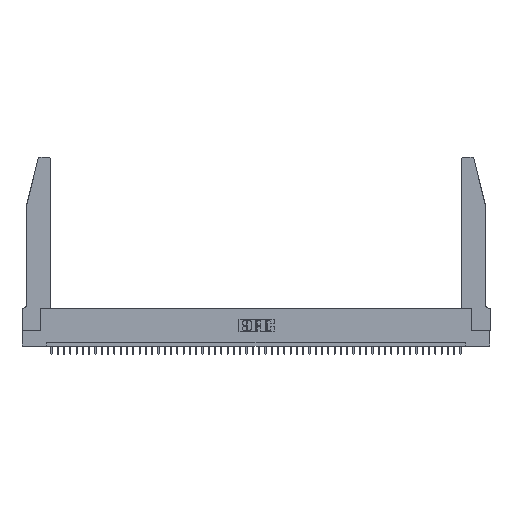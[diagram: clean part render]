
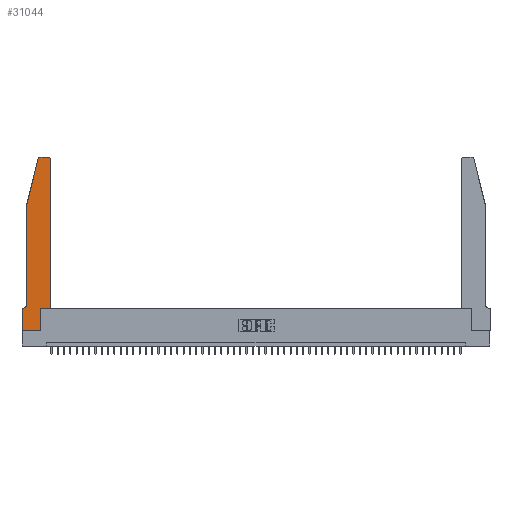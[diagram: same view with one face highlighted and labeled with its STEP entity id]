
A CAD part, top view. The second image highlights one B-rep face of the part: STEP entity #31044.
In plain terms, the highlighted planar face has unit normal (0, 0, 1).
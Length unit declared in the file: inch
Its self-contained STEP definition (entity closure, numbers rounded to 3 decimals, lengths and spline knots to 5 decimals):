
#136 = VERTEX_POINT ( 'NONE', #31626 ) ;
#412 = VECTOR ( 'NONE', #20663, 39.37008 ) ;
#1037 = ORIENTED_EDGE ( 'NONE', *, *, #36609, .T. ) ;
#2415 = CIRCLE ( 'NONE', #15642, 0.03 ) ;
#2477 = EDGE_CURVE ( 'NONE', #19180, #43705, #2415, .T. ) ;
#3498 = EDGE_LOOP ( 'NONE', ( #10704, #37596, #16229, #47534, #1037, #28264, #11088, #27232, #42411, #10031, #17437, #9026 ) ) ;
#3518 = LINE ( 'NONE', #20372, #21099 ) ;
#3726 = VERTEX_POINT ( 'NONE', #45273 ) ;
#4019 = DIRECTION ( 'NONE',  ( 0., -1., 0. ) ) ;
#5453 = AXIS2_PLACEMENT_3D ( 'NONE', #41027, #13496, #17654 ) ;
#7400 = CARTESIAN_POINT ( 'NONE',  ( 0.4505, 0.35, 0.37 ) ) ;
#7925 = DIRECTION ( 'NONE',  ( 0., 0., -1. ) ) ;
#8018 = VECTOR ( 'NONE', #47692, 39.37008 ) ;
#8240 = VERTEX_POINT ( 'NONE', #17943 ) ;
#8270 = CARTESIAN_POINT ( 'NONE',  ( 0.2865, 0.35, 0.37 ) ) ;
#8286 = DIRECTION ( 'NONE',  ( 1., 0., 0. ) ) ;
#8800 = VECTOR ( 'NONE', #20090, 39.37008 ) ;
#9026 = ORIENTED_EDGE ( 'NONE', *, *, #2477, .T. ) ;
#10031 = ORIENTED_EDGE ( 'NONE', *, *, #48210, .T. ) ;
#10631 = CARTESIAN_POINT ( 'NONE',  ( 0.0755, 0.42, 0.37 ) ) ;
#10704 = ORIENTED_EDGE ( 'NONE', *, *, #20610, .T. ) ;
#10705 = CARTESIAN_POINT ( 'NONE',  ( 0.2605, 2.75, 0.37 ) ) ;
#10942 = DIRECTION ( 'NONE',  ( -1., 0., 0. ) ) ;
#10972 = LINE ( 'NONE', #39771, #17835 ) ;
#11088 = ORIENTED_EDGE ( 'NONE', *, *, #26954, .T. ) ;
#11228 = DIRECTION ( 'NONE',  ( 1., 0., 0. ) ) ;
#12204 = AXIS2_PLACEMENT_3D ( 'NONE', #19861, #7925, #39593 ) ;
#13496 = DIRECTION ( 'NONE',  ( 0., 0., 1. ) ) ;
#15642 = AXIS2_PLACEMENT_3D ( 'NONE', #43852, #39432, #8286 ) ;
#15926 = CARTESIAN_POINT ( 'NONE',  ( 0., 0., 0.37 ) ) ;
#16121 = CARTESIAN_POINT ( 'NONE',  ( 0.0755, 2., 0.37 ) ) ;
#16218 = CARTESIAN_POINT ( 'NONE',  ( 0., 0., 0.37 ) ) ;
#16229 = ORIENTED_EDGE ( 'NONE', *, *, #16728, .T. ) ;
#16335 = CARTESIAN_POINT ( 'NONE',  ( 0.284, 2.72, 0.37 ) ) ;
#16728 = EDGE_CURVE ( 'NONE', #136, #44213, #35854, .T. ) ;
#17437 = ORIENTED_EDGE ( 'NONE', *, *, #36222, .T. ) ;
#17654 = DIRECTION ( 'NONE',  ( 1., 0., 0. ) ) ;
#17835 = VECTOR ( 'NONE', #11228, 39.37008 ) ;
#17943 = CARTESIAN_POINT ( 'NONE',  ( 0.2865, 0., 0.37 ) ) ;
#18443 = CARTESIAN_POINT ( 'NONE',  ( 0.0755, 0.35, 0.37 ) ) ;
#19180 = VERTEX_POINT ( 'NONE', #42445 ) ;
#19322 = VECTOR ( 'NONE', #31970, 39.37008 ) ;
#19861 = CARTESIAN_POINT ( 'NONE',  ( 0.0055, 0.42, 0.37 ) ) ;
#19975 = DIRECTION ( 'NONE',  ( 1., 0., 0. ) ) ;
#20090 = DIRECTION ( 'NONE',  ( 1., 0., 0. ) ) ;
#20200 = LINE ( 'NONE', #10705, #20436 ) ;
#20372 = CARTESIAN_POINT ( 'NONE',  ( 0.2865, 0.35, 0.37 ) ) ;
#20436 = VECTOR ( 'NONE', #10942, 39.37008 ) ;
#20610 = EDGE_CURVE ( 'NONE', #43705, #3726, #20200, .T. ) ;
#20663 = DIRECTION ( 'NONE',  ( 0., -1., 0. ) ) ;
#21099 = VECTOR ( 'NONE', #47619, 39.37008 ) ;
#23628 = VECTOR ( 'NONE', #4019, 39.37008 ) ;
#24652 = DIRECTION ( 'NONE',  ( 0., 0., 1. ) ) ;
#24805 = VERTEX_POINT ( 'NONE', #26966 ) ;
#24944 = VERTEX_POINT ( 'NONE', #8270 ) ;
#25740 = DIRECTION ( 'NONE',  ( -1., 0., 0. ) ) ;
#26954 = EDGE_CURVE ( 'NONE', #34084, #32753, #39567, .T. ) ;
#26966 = CARTESIAN_POINT ( 'NONE',  ( 0.0055, 0.35, 0.37 ) ) ;
#27232 = ORIENTED_EDGE ( 'NONE', *, *, #49839, .T. ) ;
#27441 = CARTESIAN_POINT ( 'NONE',  ( 0.0755, 2., 0.37 ) ) ;
#27959 = CIRCLE ( 'NONE', #12204, 0.07 ) ;
#28264 = ORIENTED_EDGE ( 'NONE', *, *, #50120, .T. ) ;
#28966 = LINE ( 'NONE', #36486, #412 ) ;
#29608 = PLANE ( 'NONE',  #5453 ) ;
#30160 = VERTEX_POINT ( 'NONE', #10631 ) ;
#30231 = EDGE_CURVE ( 'NONE', #44213, #30160, #28966, .T. ) ;
#31044 = ADVANCED_FACE ( 'NONE', ( #45686 ), #29608, .T. ) ;
#31140 = AXIS2_PLACEMENT_3D ( 'NONE', #16335, #24652, #19975 ) ;
#31626 = CARTESIAN_POINT ( 'NONE',  ( 0.25487, 2.72718, 0.37 ) ) ;
#31861 = CARTESIAN_POINT ( 'NONE',  ( 0.4505, 0.35, 0.37 ) ) ;
#31970 = DIRECTION ( 'NONE',  ( -0.239, -0.971, 0. ) ) ;
#32753 = VERTEX_POINT ( 'NONE', #16218 ) ;
#33345 = VERTEX_POINT ( 'NONE', #48860 ) ;
#34084 = VERTEX_POINT ( 'NONE', #42797 ) ;
#35425 = LINE ( 'NONE', #7400, #8800 ) ;
#35854 = LINE ( 'NONE', #16121, #19322 ) ;
#36222 = EDGE_CURVE ( 'NONE', #33345, #19180, #39653, .T. ) ;
#36486 = CARTESIAN_POINT ( 'NONE',  ( 0.0755, 2., 0.37 ) ) ;
#36609 = EDGE_CURVE ( 'NONE', #30160, #24805, #27959, .T. ) ;
#36922 = VECTOR ( 'NONE', #25740, 39.37008 ) ;
#37596 = ORIENTED_EDGE ( 'NONE', *, *, #50379, .T. ) ;
#39432 = DIRECTION ( 'NONE',  ( 0., 0., 1. ) ) ;
#39567 = LINE ( 'NONE', #15926, #23628 ) ;
#39593 = DIRECTION ( 'NONE',  ( -1., 0., 0. ) ) ;
#39653 = LINE ( 'NONE', #31861, #8018 ) ;
#39771 = CARTESIAN_POINT ( 'NONE',  ( 0., 0., 0.37 ) ) ;
#41027 = CARTESIAN_POINT ( 'NONE',  ( 0., 0.35, 0.37 ) ) ;
#42411 = ORIENTED_EDGE ( 'NONE', *, *, #50687, .T. ) ;
#42445 = CARTESIAN_POINT ( 'NONE',  ( 0.4505, 2.72, 0.37 ) ) ;
#42797 = CARTESIAN_POINT ( 'NONE',  ( 0., 0.35, 0.37 ) ) ;
#43472 = CIRCLE ( 'NONE', #31140, 0.03 ) ;
#43705 = VERTEX_POINT ( 'NONE', #45952 ) ;
#43852 = CARTESIAN_POINT ( 'NONE',  ( 0.4205, 2.72, 0.37 ) ) ;
#44213 = VERTEX_POINT ( 'NONE', #27441 ) ;
#45207 = LINE ( 'NONE', #18443, #36922 ) ;
#45273 = CARTESIAN_POINT ( 'NONE',  ( 0.284, 2.75, 0.37 ) ) ;
#45686 = FACE_OUTER_BOUND ( 'NONE', #3498, .T. ) ;
#45952 = CARTESIAN_POINT ( 'NONE',  ( 0.4205, 2.75, 0.37 ) ) ;
#47534 = ORIENTED_EDGE ( 'NONE', *, *, #30231, .T. ) ;
#47619 = DIRECTION ( 'NONE',  ( 0., 1., 0. ) ) ;
#47692 = DIRECTION ( 'NONE',  ( 0., 1., 0. ) ) ;
#48210 = EDGE_CURVE ( 'NONE', #24944, #33345, #35425, .T. ) ;
#48860 = CARTESIAN_POINT ( 'NONE',  ( 0.4505, 0.35, 0.37 ) ) ;
#49839 = EDGE_CURVE ( 'NONE', #32753, #8240, #10972, .T. ) ;
#50120 = EDGE_CURVE ( 'NONE', #24805, #34084, #45207, .T. ) ;
#50379 = EDGE_CURVE ( 'NONE', #3726, #136, #43472, .T. ) ;
#50687 = EDGE_CURVE ( 'NONE', #8240, #24944, #3518, .T. ) ;
